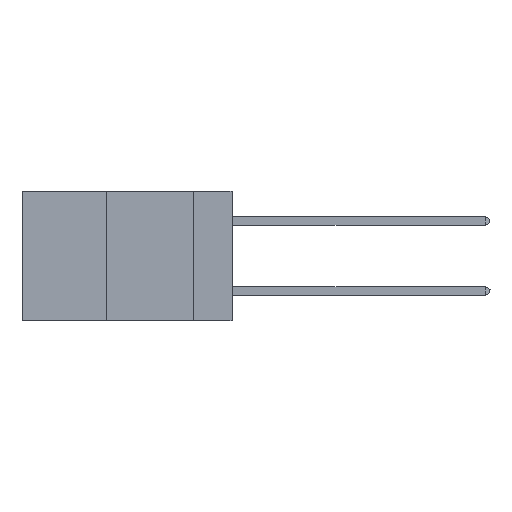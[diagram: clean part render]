
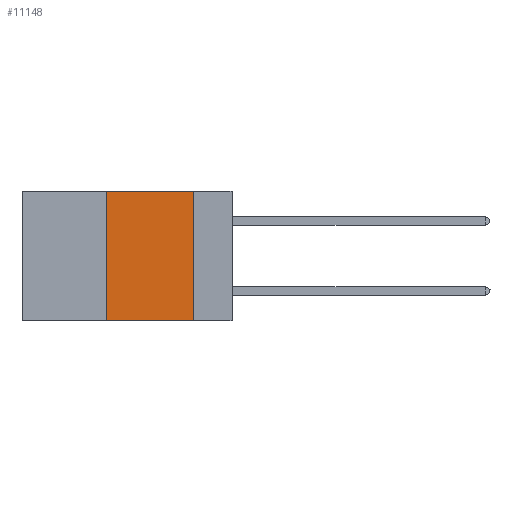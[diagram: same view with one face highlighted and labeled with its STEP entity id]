
A CAD part, left-side view. The second image highlights one B-rep face of the part: STEP entity #11148.
In plain terms, the highlighted planar face has unit normal (-1, 0, 0).
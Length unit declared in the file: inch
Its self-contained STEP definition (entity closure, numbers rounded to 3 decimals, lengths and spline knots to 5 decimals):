
#1895 = ORIENTED_EDGE ( 'NONE', *, *, #16834, .F. ) ;
#2122 = EDGE_CURVE ( 'NONE', #16273, #12106, #6376, .T. ) ;
#2329 = VECTOR ( 'NONE', #18084, 39.37008 ) ;
#2611 = EDGE_CURVE ( 'NONE', #6540, #12106, #15603, .T. ) ;
#3492 = CARTESIAN_POINT ( 'NONE',  ( 0., 0.6, -0.37 ) ) ;
#3746 = PLANE ( 'NONE',  #7710 ) ;
#3926 = LINE ( 'NONE', #15986, #19252 ) ;
#3928 = CARTESIAN_POINT ( 'NONE',  ( 0., 0.11, 0. ) ) ;
#3957 = DIRECTION ( 'NONE',  ( 0., -1., 0. ) ) ;
#4333 = ORIENTED_EDGE ( 'NONE', *, *, #17636, .F. ) ;
#6376 = LINE ( 'NONE', #3492, #2329 ) ;
#6540 = VERTEX_POINT ( 'NONE', #3928 ) ;
#7710 = AXIS2_PLACEMENT_3D ( 'NONE', #16751, #12780, #14249 ) ;
#8288 = ORIENTED_EDGE ( 'NONE', *, *, #2122, .T. ) ;
#9104 = CARTESIAN_POINT ( 'NONE',  ( 0., 0.36, 0. ) ) ;
#10005 = LINE ( 'NONE', #15883, #13516 ) ;
#11148 = ADVANCED_FACE ( 'NONE', ( #14014 ), #3746, .F. ) ;
#12106 = VERTEX_POINT ( 'NONE', #15371 ) ;
#12258 = VERTEX_POINT ( 'NONE', #9104 ) ;
#12780 = DIRECTION ( 'NONE',  ( 1., 0., 0. ) ) ;
#13109 = DIRECTION ( 'NONE',  ( 0., 0., 1. ) ) ;
#13516 = VECTOR ( 'NONE', #3957, 39.37008 ) ;
#14014 = FACE_OUTER_BOUND ( 'NONE', #14290, .T. ) ;
#14249 = DIRECTION ( 'NONE',  ( 0., 0., -1. ) ) ;
#14290 = EDGE_LOOP ( 'NONE', ( #17691, #1895, #4333, #8288 ) ) ;
#15355 = CARTESIAN_POINT ( 'NONE',  ( 0., 0.11, 0. ) ) ;
#15371 = CARTESIAN_POINT ( 'NONE',  ( 0., 0.11, -0.37 ) ) ;
#15603 = LINE ( 'NONE', #15355, #15823 ) ;
#15645 = CARTESIAN_POINT ( 'NONE',  ( 0., 0.36, -0.37 ) ) ;
#15823 = VECTOR ( 'NONE', #17962, 39.37008 ) ;
#15883 = CARTESIAN_POINT ( 'NONE',  ( 0., 0.6, 0. ) ) ;
#15986 = CARTESIAN_POINT ( 'NONE',  ( 0., 0.36, 0. ) ) ;
#16273 = VERTEX_POINT ( 'NONE', #15645 ) ;
#16751 = CARTESIAN_POINT ( 'NONE',  ( 0., 0.6, 0. ) ) ;
#16834 = EDGE_CURVE ( 'NONE', #12258, #6540, #10005, .T. ) ;
#17636 = EDGE_CURVE ( 'NONE', #16273, #12258, #3926, .T. ) ;
#17691 = ORIENTED_EDGE ( 'NONE', *, *, #2611, .F. ) ;
#17962 = DIRECTION ( 'NONE',  ( 0., 0., -1. ) ) ;
#18084 = DIRECTION ( 'NONE',  ( 0., -1., 0. ) ) ;
#19252 = VECTOR ( 'NONE', #13109, 39.37008 ) ;
